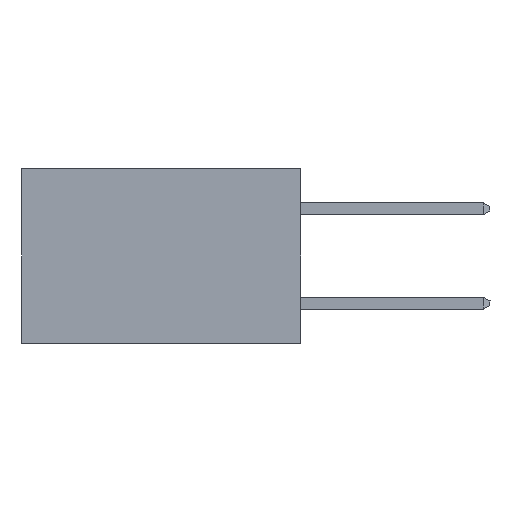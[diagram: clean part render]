
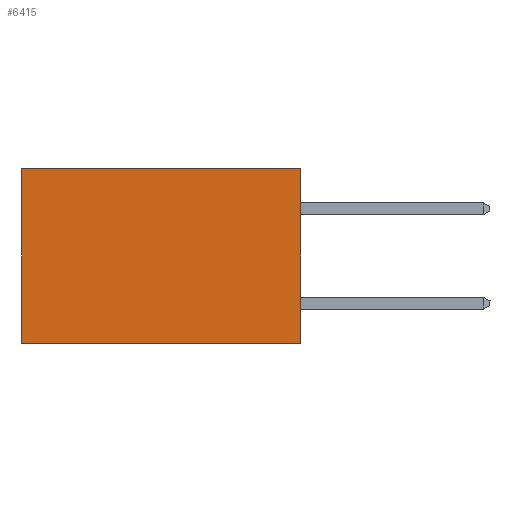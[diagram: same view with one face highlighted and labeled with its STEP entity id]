
A CAD part, left-side view. The second image highlights one B-rep face of the part: STEP entity #6415.
In plain terms, the highlighted planar face has unit normal (-1, 0, 0).
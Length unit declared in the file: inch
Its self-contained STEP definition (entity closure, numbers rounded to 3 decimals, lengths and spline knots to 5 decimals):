
#280 = CARTESIAN_POINT ( 'NONE',  ( 0.277, 0.59, 0. ) ) ;
#537 = FACE_OUTER_BOUND ( 'NONE', #9361, .T. ) ;
#917 = EDGE_CURVE ( 'NONE', #8924, #6279, #3922, .T. ) ;
#985 = ORIENTED_EDGE ( 'NONE', *, *, #9160, .T. ) ;
#1015 = CARTESIAN_POINT ( 'NONE',  ( 0.277, 0., -0.37 ) ) ;
#1157 = CARTESIAN_POINT ( 'NONE',  ( 0.277, 0., 0. ) ) ;
#1239 = ORIENTED_EDGE ( 'NONE', *, *, #2742, .F. ) ;
#1240 = DIRECTION ( 'NONE',  ( 0., 0., -1. ) ) ;
#1356 = ORIENTED_EDGE ( 'NONE', *, *, #2763, .F. ) ;
#1433 = ORIENTED_EDGE ( 'NONE', *, *, #917, .T. ) ;
#2626 = DIRECTION ( 'NONE',  ( 0., 1., 0. ) ) ;
#2678 = CARTESIAN_POINT ( 'NONE',  ( 0.277, 0., -0.37 ) ) ;
#2742 = EDGE_CURVE ( 'NONE', #6366, #5270, #8888, .T. ) ;
#2762 = VECTOR ( 'NONE', #1240, 39.37008 ) ;
#2763 = EDGE_CURVE ( 'NONE', #8924, #6366, #8474, .T. ) ;
#2935 = DIRECTION ( 'NONE',  ( 0., 0., -1. ) ) ;
#3248 = VECTOR ( 'NONE', #2626, 39.37008 ) ;
#3922 = LINE ( 'NONE', #1157, #9023 ) ;
#4401 = LINE ( 'NONE', #8605, #9233 ) ;
#5270 = VERTEX_POINT ( 'NONE', #9302 ) ;
#5799 = CARTESIAN_POINT ( 'NONE',  ( 0.277, 0., 0. ) ) ;
#5944 = DIRECTION ( 'NONE',  ( 0., 0., -1. ) ) ;
#6127 = DIRECTION ( 'NONE',  ( 1., 0., 0. ) ) ;
#6132 = CARTESIAN_POINT ( 'NONE',  ( 0.277, 0., -0.37 ) ) ;
#6279 = VERTEX_POINT ( 'NONE', #280 ) ;
#6366 = VERTEX_POINT ( 'NONE', #8458 ) ;
#6415 = ADVANCED_FACE ( 'NONE', ( #537 ), #6511, .F. ) ;
#6511 = PLANE ( 'NONE',  #7005 ) ;
#7005 = AXIS2_PLACEMENT_3D ( 'NONE', #6132, #6127, #5944 ) ;
#7723 = DIRECTION ( 'NONE',  ( 0., 1., 0. ) ) ;
#8458 = CARTESIAN_POINT ( 'NONE',  ( 0.277, 0., -0.37 ) ) ;
#8474 = LINE ( 'NONE', #1015, #2762 ) ;
#8605 = CARTESIAN_POINT ( 'NONE',  ( 0.277, 0.59, -0.37 ) ) ;
#8888 = LINE ( 'NONE', #2678, #3248 ) ;
#8924 = VERTEX_POINT ( 'NONE', #5799 ) ;
#9023 = VECTOR ( 'NONE', #7723, 39.37008 ) ;
#9160 = EDGE_CURVE ( 'NONE', #6279, #5270, #4401, .T. ) ;
#9233 = VECTOR ( 'NONE', #2935, 39.37008 ) ;
#9302 = CARTESIAN_POINT ( 'NONE',  ( 0.277, 0.59, -0.37 ) ) ;
#9361 = EDGE_LOOP ( 'NONE', ( #985, #1239, #1356, #1433 ) ) ;
